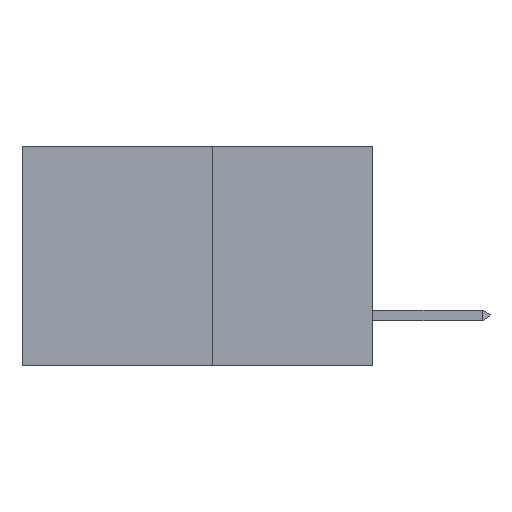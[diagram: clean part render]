
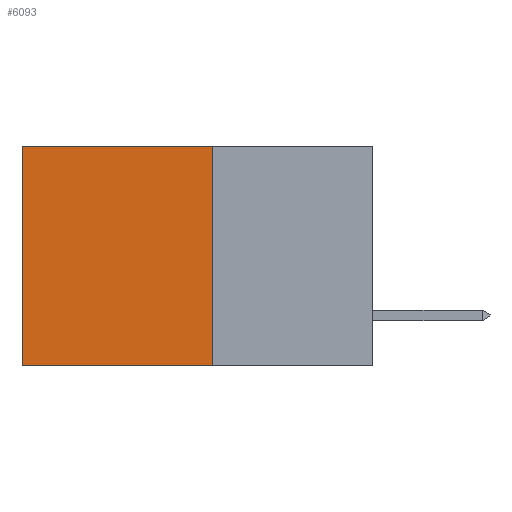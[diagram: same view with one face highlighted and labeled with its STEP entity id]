
A CAD part, left-side view. The second image highlights one B-rep face of the part: STEP entity #6093.
In plain terms, the highlighted planar face has unit normal (-1, 0, 0).
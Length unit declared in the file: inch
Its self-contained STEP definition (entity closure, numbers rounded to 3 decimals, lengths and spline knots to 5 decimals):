
#30 = PLANE ( 'NONE',  #5317 ) ;
#82 = CARTESIAN_POINT ( 'NONE',  ( 0.277, 0.27, 0. ) ) ;
#787 = LINE ( 'NONE', #5389, #11067 ) ;
#1050 = DIRECTION ( 'NONE',  ( 0., 1., 0. ) ) ;
#1394 = VERTEX_POINT ( 'NONE', #7207 ) ;
#1416 = CARTESIAN_POINT ( 'NONE',  ( 0.277, 0.59, 0. ) ) ;
#2124 = LINE ( 'NONE', #4584, #10057 ) ;
#2145 = EDGE_CURVE ( 'NONE', #9097, #5189, #9443, .T. ) ;
#2542 = EDGE_CURVE ( 'NONE', #9283, #1394, #2124, .T. ) ;
#3046 = EDGE_CURVE ( 'NONE', #5189, #1394, #787, .T. ) ;
#3066 = DIRECTION ( 'NONE',  ( 1., 0., 0. ) ) ;
#4092 = ORIENTED_EDGE ( 'NONE', *, *, #9751, .T. ) ;
#4121 = ORIENTED_EDGE ( 'NONE', *, *, #3046, .F. ) ;
#4144 = VECTOR ( 'NONE', #4816, 39.37008 ) ;
#4443 = EDGE_LOOP ( 'NONE', ( #11642, #4121, #10135, #4092 ) ) ;
#4584 = CARTESIAN_POINT ( 'NONE',  ( 0.277, 0.59, -0.37 ) ) ;
#4816 = DIRECTION ( 'NONE',  ( 0., 0., -1. ) ) ;
#5189 = VERTEX_POINT ( 'NONE', #8647 ) ;
#5317 = AXIS2_PLACEMENT_3D ( 'NONE', #9540, #3066, #10037 ) ;
#5370 = FACE_OUTER_BOUND ( 'NONE', #4443, .T. ) ;
#5389 = CARTESIAN_POINT ( 'NONE',  ( 0.277, 0.27, -0.37 ) ) ;
#6093 = ADVANCED_FACE ( 'NONE', ( #5370 ), #30, .F. ) ;
#7207 = CARTESIAN_POINT ( 'NONE',  ( 0.277, 0.59, -0.37 ) ) ;
#7459 = LINE ( 'NONE', #10954, #12418 ) ;
#8647 = CARTESIAN_POINT ( 'NONE',  ( 0.277, 0.27, -0.37 ) ) ;
#8777 = CARTESIAN_POINT ( 'NONE',  ( 0.277, 0.27, -0.37 ) ) ;
#9097 = VERTEX_POINT ( 'NONE', #82 ) ;
#9283 = VERTEX_POINT ( 'NONE', #1416 ) ;
#9443 = LINE ( 'NONE', #8777, #4144 ) ;
#9540 = CARTESIAN_POINT ( 'NONE',  ( 0.277, 0.27, -0.37 ) ) ;
#9751 = EDGE_CURVE ( 'NONE', #9097, #9283, #7459, .T. ) ;
#10037 = DIRECTION ( 'NONE',  ( 0., 0., -1. ) ) ;
#10057 = VECTOR ( 'NONE', #10551, 39.37008 ) ;
#10135 = ORIENTED_EDGE ( 'NONE', *, *, #2145, .F. ) ;
#10551 = DIRECTION ( 'NONE',  ( 0., 0., -1. ) ) ;
#10954 = CARTESIAN_POINT ( 'NONE',  ( 0.277, 0.27, 0. ) ) ;
#11067 = VECTOR ( 'NONE', #11343, 39.37008 ) ;
#11343 = DIRECTION ( 'NONE',  ( 0., 1., 0. ) ) ;
#11642 = ORIENTED_EDGE ( 'NONE', *, *, #2542, .T. ) ;
#12418 = VECTOR ( 'NONE', #1050, 39.37008 ) ;
